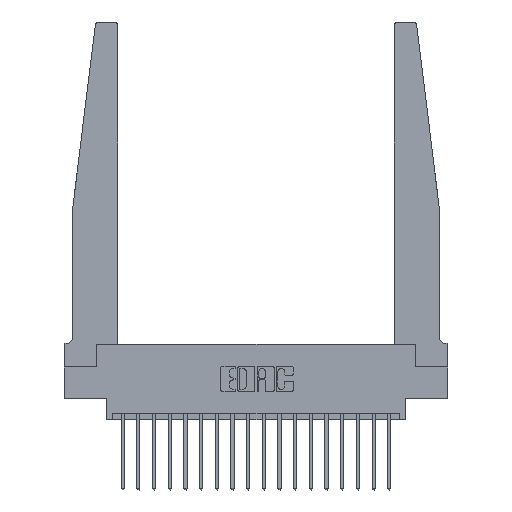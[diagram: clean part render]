
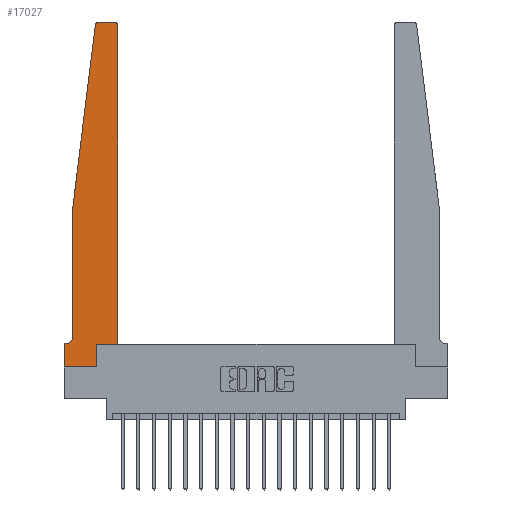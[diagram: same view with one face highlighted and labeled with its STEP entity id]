
A CAD part, top view. The second image highlights one B-rep face of the part: STEP entity #17027.
In plain terms, the highlighted planar face has unit normal (0, 0, 1).
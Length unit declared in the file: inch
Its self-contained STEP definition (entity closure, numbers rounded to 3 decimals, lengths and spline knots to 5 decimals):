
#486 = ORIENTED_EDGE ( 'NONE', *, *, #14313, .T. ) ;
#594 = CARTESIAN_POINT ( 'NONE',  ( 0.425, 0.18, 0.37 ) ) ;
#762 = LINE ( 'NONE', #18156, #8728 ) ;
#785 = DIRECTION ( 'NONE',  ( 1., 0., 0. ) ) ;
#924 = EDGE_LOOP ( 'NONE', ( #11183, #14949, #4271, #12134, #4248, #2588, #10918, #17372, #2809, #18291, #5739, #486 ) ) ;
#1369 = CARTESIAN_POINT ( 'NONE',  ( 0., 0., 0.37 ) ) ;
#2110 = VERTEX_POINT ( 'NONE', #12165 ) ;
#2315 = DIRECTION ( 'NONE',  ( 0., 0., 1. ) ) ;
#2437 = LINE ( 'NONE', #16509, #13196 ) ;
#2588 = ORIENTED_EDGE ( 'NONE', *, *, #19753, .T. ) ;
#2613 = LINE ( 'NONE', #9731, #14781 ) ;
#2626 = CIRCLE ( 'NONE', #13119, 0.03 ) ;
#2809 = ORIENTED_EDGE ( 'NONE', *, *, #4295, .T. ) ;
#3009 = VERTEX_POINT ( 'NONE', #8643 ) ;
#3072 = EDGE_CURVE ( 'NONE', #17824, #12271, #10084, .T. ) ;
#3344 = EDGE_CURVE ( 'NONE', #12372, #3009, #15101, .T. ) ;
#4096 = DIRECTION ( 'NONE',  ( 1., 0., 0. ) ) ;
#4220 = CARTESIAN_POINT ( 'NONE',  ( 0.015, 0.2375, 0.37 ) ) ;
#4248 = ORIENTED_EDGE ( 'NONE', *, *, #19531, .T. ) ;
#4271 = ORIENTED_EDGE ( 'NONE', *, *, #5066, .T. ) ;
#4295 = EDGE_CURVE ( 'NONE', #2110, #12042, #13191, .T. ) ;
#4748 = CARTESIAN_POINT ( 'NONE',  ( 0.25, 2.75, 0.37 ) ) ;
#5066 = EDGE_CURVE ( 'NONE', #3009, #17824, #762, .T. ) ;
#5481 = DIRECTION ( 'NONE',  ( 0., 1., 0. ) ) ;
#5557 = VERTEX_POINT ( 'NONE', #9913 ) ;
#5566 = DIRECTION ( 'NONE',  ( 0., 0., 1. ) ) ;
#5694 = VECTOR ( 'NONE', #6567, 39.37008 ) ;
#5739 = ORIENTED_EDGE ( 'NONE', *, *, #15205, .T. ) ;
#5824 = DIRECTION ( 'NONE',  ( 1., 0., 0. ) ) ;
#6567 = DIRECTION ( 'NONE',  ( -1., 0., 0. ) ) ;
#6695 = AXIS2_PLACEMENT_3D ( 'NONE', #8834, #5566, #785 ) ;
#6914 = DIRECTION ( 'NONE',  ( 0., -1., 0. ) ) ;
#6919 = CARTESIAN_POINT ( 'NONE',  ( 0.065, 1.25, 0.37 ) ) ;
#6999 = VECTOR ( 'NONE', #13679, 39.37008 ) ;
#7054 = CARTESIAN_POINT ( 'NONE',  ( 0.2605, 0.18, 0.37 ) ) ;
#7330 = CARTESIAN_POINT ( 'NONE',  ( 0.425, 2.72, 0.37 ) ) ;
#8199 = DIRECTION ( 'NONE',  ( 0., -1., 0. ) ) ;
#8235 = VERTEX_POINT ( 'NONE', #13938 ) ;
#8306 = CIRCLE ( 'NONE', #20117, 0.05 ) ;
#8643 = CARTESIAN_POINT ( 'NONE',  ( 0.24675, 2.72367, 0.37 ) ) ;
#8728 = VECTOR ( 'NONE', #16502, 39.37008 ) ;
#8834 = CARTESIAN_POINT ( 'NONE',  ( 0.27653, 2.72, 0.37 ) ) ;
#8935 = DIRECTION ( 'NONE',  ( 1., 0., 0. ) ) ;
#8959 = CARTESIAN_POINT ( 'NONE',  ( 0.065, 1.25, 0.37 ) ) ;
#9016 = VERTEX_POINT ( 'NONE', #9372 ) ;
#9217 = AXIS2_PLACEMENT_3D ( 'NONE', #19734, #18578, #8935 ) ;
#9372 = CARTESIAN_POINT ( 'NONE',  ( 0., 0., 0.37 ) ) ;
#9645 = LINE ( 'NONE', #4748, #5694 ) ;
#9731 = CARTESIAN_POINT ( 'NONE',  ( 0., 0., 0.37 ) ) ;
#9913 = CARTESIAN_POINT ( 'NONE',  ( 0.015, 0.1875, 0.37 ) ) ;
#10084 = LINE ( 'NONE', #8959, #13675 ) ;
#10466 = DIRECTION ( 'NONE',  ( -1., 0., 0. ) ) ;
#10750 = CARTESIAN_POINT ( 'NONE',  ( 0.2605, 0.18, 0.37 ) ) ;
#10918 = ORIENTED_EDGE ( 'NONE', *, *, #17356, .T. ) ;
#11183 = ORIENTED_EDGE ( 'NONE', *, *, #19157, .T. ) ;
#11564 = CARTESIAN_POINT ( 'NONE',  ( 0.065, 0.2375, 0.37 ) ) ;
#11577 = CARTESIAN_POINT ( 'NONE',  ( 0.395, 2.72, 0.37 ) ) ;
#11773 = VERTEX_POINT ( 'NONE', #7330 ) ;
#12042 = VERTEX_POINT ( 'NONE', #10750 ) ;
#12122 = FACE_OUTER_BOUND ( 'NONE', #924, .T. ) ;
#12134 = ORIENTED_EDGE ( 'NONE', *, *, #3072, .T. ) ;
#12165 = CARTESIAN_POINT ( 'NONE',  ( 0.2605, 0., 0.37 ) ) ;
#12271 = VERTEX_POINT ( 'NONE', #11564 ) ;
#12372 = VERTEX_POINT ( 'NONE', #17082 ) ;
#13049 = LINE ( 'NONE', #16132, #20051 ) ;
#13119 = AXIS2_PLACEMENT_3D ( 'NONE', #11577, #2315, #4096 ) ;
#13191 = LINE ( 'NONE', #7054, #18866 ) ;
#13196 = VECTOR ( 'NONE', #16614, 39.37008 ) ;
#13550 = PLANE ( 'NONE',  #9217 ) ;
#13675 = VECTOR ( 'NONE', #6914, 39.37008 ) ;
#13679 = DIRECTION ( 'NONE',  ( -1., 0., 0. ) ) ;
#13822 = VECTOR ( 'NONE', #5824, 39.37008 ) ;
#13938 = CARTESIAN_POINT ( 'NONE',  ( 0., 0.1875, 0.37 ) ) ;
#14313 = EDGE_CURVE ( 'NONE', #11773, #16276, #2626, .T. ) ;
#14781 = VECTOR ( 'NONE', #8199, 39.37008 ) ;
#14949 = ORIENTED_EDGE ( 'NONE', *, *, #3344, .T. ) ;
#15101 = CIRCLE ( 'NONE', #6695, 0.03 ) ;
#15205 = EDGE_CURVE ( 'NONE', #20085, #11773, #13049, .T. ) ;
#16132 = CARTESIAN_POINT ( 'NONE',  ( 0.425, 0.18, 0.37 ) ) ;
#16276 = VERTEX_POINT ( 'NONE', #18830 ) ;
#16502 = DIRECTION ( 'NONE',  ( -0.122, -0.992, 0. ) ) ;
#16509 = CARTESIAN_POINT ( 'NONE',  ( 0.425, 0.18, 0.37 ) ) ;
#16614 = DIRECTION ( 'NONE',  ( 1., 0., 0. ) ) ;
#17027 = ADVANCED_FACE ( 'NONE', ( #12122 ), #13550, .T. ) ;
#17082 = CARTESIAN_POINT ( 'NONE',  ( 0.27653, 2.75, 0.37 ) ) ;
#17356 = EDGE_CURVE ( 'NONE', #8235, #9016, #2613, .T. ) ;
#17372 = ORIENTED_EDGE ( 'NONE', *, *, #17536, .T. ) ;
#17536 = EDGE_CURVE ( 'NONE', #9016, #2110, #19890, .T. ) ;
#17702 = DIRECTION ( 'NONE',  ( 0., 1., 0. ) ) ;
#17824 = VERTEX_POINT ( 'NONE', #6919 ) ;
#18111 = LINE ( 'NONE', #18316, #6999 ) ;
#18156 = CARTESIAN_POINT ( 'NONE',  ( 0.065, 1.25, 0.37 ) ) ;
#18291 = ORIENTED_EDGE ( 'NONE', *, *, #19352, .T. ) ;
#18316 = CARTESIAN_POINT ( 'NONE',  ( 0.065, 0.1875, 0.37 ) ) ;
#18578 = DIRECTION ( 'NONE',  ( 0., 0., 1. ) ) ;
#18830 = CARTESIAN_POINT ( 'NONE',  ( 0.395, 2.75, 0.37 ) ) ;
#18866 = VECTOR ( 'NONE', #17702, 39.37008 ) ;
#19157 = EDGE_CURVE ( 'NONE', #16276, #12372, #9645, .T. ) ;
#19352 = EDGE_CURVE ( 'NONE', #12042, #20085, #2437, .T. ) ;
#19531 = EDGE_CURVE ( 'NONE', #12271, #5557, #8306, .T. ) ;
#19734 = CARTESIAN_POINT ( 'NONE',  ( 0., 0.1875, 0.37 ) ) ;
#19753 = EDGE_CURVE ( 'NONE', #5557, #8235, #18111, .T. ) ;
#19890 = LINE ( 'NONE', #1369, #13822 ) ;
#20051 = VECTOR ( 'NONE', #5481, 39.37008 ) ;
#20085 = VERTEX_POINT ( 'NONE', #594 ) ;
#20117 = AXIS2_PLACEMENT_3D ( 'NONE', #4220, #20214, #10466 ) ;
#20214 = DIRECTION ( 'NONE',  ( 0., 0., -1. ) ) ;
